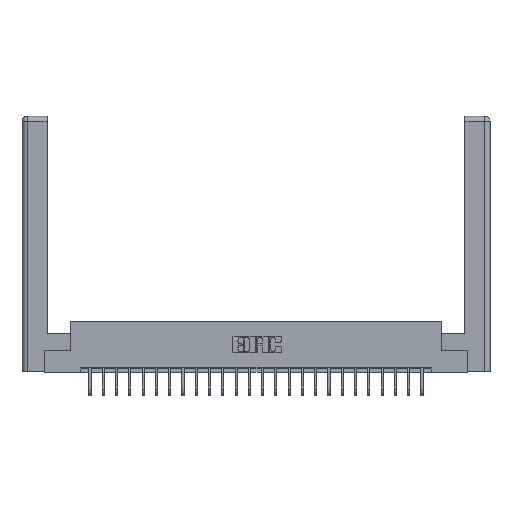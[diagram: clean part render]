
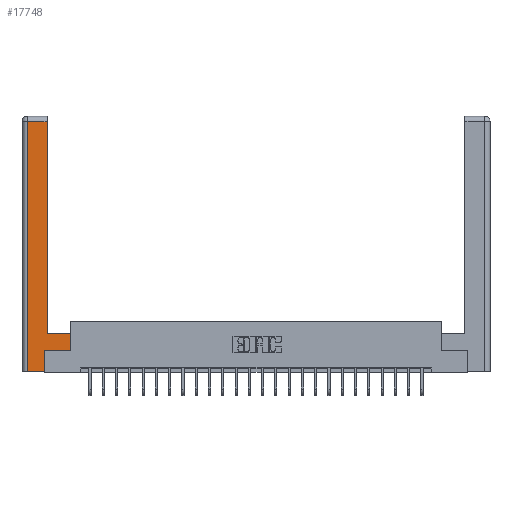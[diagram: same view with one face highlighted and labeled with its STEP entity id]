
A CAD part, top view. The second image highlights one B-rep face of the part: STEP entity #17748.
In plain terms, the highlighted planar face has unit normal (0, 0, 1).
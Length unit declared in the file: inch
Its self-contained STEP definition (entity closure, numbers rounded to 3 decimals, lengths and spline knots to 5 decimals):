
#168 = CARTESIAN_POINT ( 'NONE',  ( 0.295, 0.45, 0. ) ) ;
#357 = ORIENTED_EDGE ( 'NONE', *, *, #21700, .T. ) ;
#1083 = DIRECTION ( 'NONE',  ( 1., 0., 0. ) ) ;
#1180 = CARTESIAN_POINT ( 'NONE',  ( 0.565, 0.245, 0. ) ) ;
#1425 = VECTOR ( 'NONE', #10589, 39.37008 ) ;
#1744 = EDGE_CURVE ( 'NONE', #14883, #11520, #12983, .T. ) ;
#2041 = LINE ( 'NONE', #168, #2692 ) ;
#2203 = CARTESIAN_POINT ( 'NONE',  ( 0.265, 0., 0. ) ) ;
#2242 = CARTESIAN_POINT ( 'NONE',  ( 0.0615, 0., 0. ) ) ;
#2435 = CARTESIAN_POINT ( 'NONE',  ( 0.0615, 2.94, 0. ) ) ;
#2692 = VECTOR ( 'NONE', #14770, 39.37008 ) ;
#3050 = CARTESIAN_POINT ( 'NONE',  ( 0.565, 0.245, 0. ) ) ;
#3933 = VERTEX_POINT ( 'NONE', #2435 ) ;
#4725 = LINE ( 'NONE', #5013, #25312 ) ;
#4986 = VERTEX_POINT ( 'NONE', #2242 ) ;
#5013 = CARTESIAN_POINT ( 'NONE',  ( 0.0615, 0., 0. ) ) ;
#5090 = ORIENTED_EDGE ( 'NONE', *, *, #18178, .T. ) ;
#5361 = LINE ( 'NONE', #11655, #23407 ) ;
#6036 = VECTOR ( 'NONE', #8053, 39.37008 ) ;
#6464 = LINE ( 'NONE', #12575, #14538 ) ;
#6679 = LINE ( 'NONE', #20387, #6036 ) ;
#7387 = EDGE_CURVE ( 'NONE', #4986, #7883, #5361, .T. ) ;
#7883 = VERTEX_POINT ( 'NONE', #2203 ) ;
#8053 = DIRECTION ( 'NONE',  ( 0., 1., 0. ) ) ;
#8222 = ORIENTED_EDGE ( 'NONE', *, *, #9757, .T. ) ;
#8437 = ORIENTED_EDGE ( 'NONE', *, *, #11329, .T. ) ;
#9546 = CARTESIAN_POINT ( 'NONE',  ( 0., 0., 0. ) ) ;
#9757 = EDGE_CURVE ( 'NONE', #9979, #14608, #2041, .T. ) ;
#9979 = VERTEX_POINT ( 'NONE', #20823 ) ;
#10184 = EDGE_LOOP ( 'NONE', ( #357, #8437, #21385, #16680, #5090, #14694, #21704, #8222 ) ) ;
#10589 = DIRECTION ( 'NONE',  ( 0., 1., 0. ) ) ;
#11275 = CARTESIAN_POINT ( 'NONE',  ( 0.265, 0.245, 0. ) ) ;
#11329 = EDGE_CURVE ( 'NONE', #17984, #3933, #12225, .T. ) ;
#11520 = VERTEX_POINT ( 'NONE', #1180 ) ;
#11622 = DIRECTION ( 'NONE',  ( -1., 0., 0. ) ) ;
#11655 = CARTESIAN_POINT ( 'NONE',  ( 0.265, 0., 0. ) ) ;
#11880 = EDGE_CURVE ( 'NONE', #3933, #4986, #4725, .T. ) ;
#12225 = LINE ( 'NONE', #15087, #12568 ) ;
#12568 = VECTOR ( 'NONE', #21735, 39.37008 ) ;
#12575 = CARTESIAN_POINT ( 'NONE',  ( 0.295, 3., 0. ) ) ;
#12983 = LINE ( 'NONE', #3050, #22331 ) ;
#13015 = LINE ( 'NONE', #17917, #1425 ) ;
#14538 = VECTOR ( 'NONE', #18794, 39.37008 ) ;
#14608 = VERTEX_POINT ( 'NONE', #22932 ) ;
#14694 = ORIENTED_EDGE ( 'NONE', *, *, #1744, .T. ) ;
#14770 = DIRECTION ( 'NONE',  ( -1., 0., 0. ) ) ;
#14883 = VERTEX_POINT ( 'NONE', #11275 ) ;
#15087 = CARTESIAN_POINT ( 'NONE',  ( 0.0615, 2.94, 0. ) ) ;
#16680 = ORIENTED_EDGE ( 'NONE', *, *, #7387, .T. ) ;
#17675 = DIRECTION ( 'NONE',  ( 0., 0., -1. ) ) ;
#17748 = ADVANCED_FACE ( 'NONE', ( #18164 ), #23683, .F. ) ;
#17917 = CARTESIAN_POINT ( 'NONE',  ( 0.265, 0.245, 0. ) ) ;
#17984 = VERTEX_POINT ( 'NONE', #24942 ) ;
#18164 = FACE_OUTER_BOUND ( 'NONE', #10184, .T. ) ;
#18178 = EDGE_CURVE ( 'NONE', #7883, #14883, #13015, .T. ) ;
#18794 = DIRECTION ( 'NONE',  ( 0., 1., 0. ) ) ;
#20387 = CARTESIAN_POINT ( 'NONE',  ( 0.565, 0.45, 0. ) ) ;
#20823 = CARTESIAN_POINT ( 'NONE',  ( 0.565, 0.45, 0. ) ) ;
#21385 = ORIENTED_EDGE ( 'NONE', *, *, #11880, .T. ) ;
#21700 = EDGE_CURVE ( 'NONE', #14608, #17984, #6464, .T. ) ;
#21704 = ORIENTED_EDGE ( 'NONE', *, *, #25453, .T. ) ;
#21735 = DIRECTION ( 'NONE',  ( -1., 0., 0. ) ) ;
#22331 = VECTOR ( 'NONE', #1083, 39.37008 ) ;
#22932 = CARTESIAN_POINT ( 'NONE',  ( 0.295, 0.45, 0. ) ) ;
#23407 = VECTOR ( 'NONE', #25898, 39.37008 ) ;
#23627 = DIRECTION ( 'NONE',  ( 0., -1., 0. ) ) ;
#23683 = PLANE ( 'NONE',  #23890 ) ;
#23890 = AXIS2_PLACEMENT_3D ( 'NONE', #9546, #17675, #11622 ) ;
#24942 = CARTESIAN_POINT ( 'NONE',  ( 0.295, 2.94, 0. ) ) ;
#25312 = VECTOR ( 'NONE', #23627, 39.37008 ) ;
#25453 = EDGE_CURVE ( 'NONE', #11520, #9979, #6679, .T. ) ;
#25898 = DIRECTION ( 'NONE',  ( 1., 0., 0. ) ) ;
